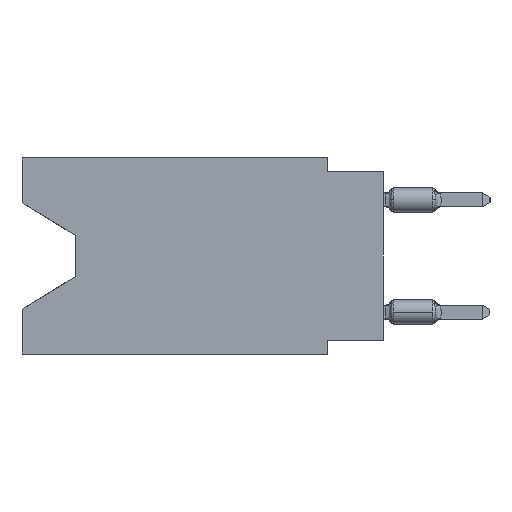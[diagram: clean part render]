
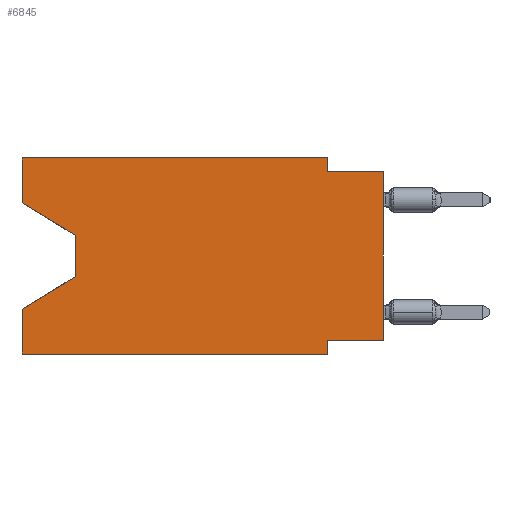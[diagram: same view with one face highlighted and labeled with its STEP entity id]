
A CAD part, left-side view. The second image highlights one B-rep face of the part: STEP entity #6845.
In plain terms, the highlighted planar face has unit normal (-1, 0, 0).
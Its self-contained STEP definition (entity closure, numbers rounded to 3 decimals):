
#188 = CARTESIAN_POINT ( 'NONE',  ( 0., 16.383, 0. ) ) ;
#1054 = CARTESIAN_POINT ( 'NONE',  ( 0., 2.54, 0. ) ) ;
#1588 = VERTEX_POINT ( 'NONE', #1054 ) ;
#1661 = VERTEX_POINT ( 'NONE', #5402 ) ;
#2791 = DIRECTION ( 'NONE',  ( 0., 0., 1. ) ) ;
#3307 = CARTESIAN_POINT ( 'NONE',  ( 0., 16.383, 0. ) ) ;
#3819 = LINE ( 'NONE', #188, #11470 ) ;
#4029 = CARTESIAN_POINT ( 'NONE',  ( 0., 16.383, 0. ) ) ;
#5402 = CARTESIAN_POINT ( 'NONE',  ( 0., 16.383, -8.89 ) ) ;
#5623 = CARTESIAN_POINT ( 'NONE',  ( 0., 16.383, -6.852 ) ) ;
#6257 = EDGE_CURVE ( 'NONE', #7869, #8992, #46836, .T. ) ;
#6414 = CARTESIAN_POINT ( 'NONE',  ( 0., 13.97, -5.385 ) ) ;
#6783 = DIRECTION ( 'NONE',  ( 0., 0., 1. ) ) ;
#6845 = ADVANCED_FACE ( 'NONE', ( #30512 ), #23268, .F. ) ;
#7869 = VERTEX_POINT ( 'NONE', #35128 ) ;
#8992 = VERTEX_POINT ( 'NONE', #31027 ) ;
#9885 = EDGE_LOOP ( 'NONE', ( #32290, #25213, #33541, #35533, #13075, #37361, #36365, #41042, #34936, #41778, #25624, #45189 ) ) ;
#9987 = EDGE_CURVE ( 'NONE', #44890, #39146, #24137, .T. ) ;
#10009 = VECTOR ( 'NONE', #6783, 1000. ) ;
#10449 = EDGE_CURVE ( 'NONE', #46667, #24446, #29289, .T. ) ;
#10716 = CARTESIAN_POINT ( 'NONE',  ( 0., 13.97, -5.385 ) ) ;
#11265 = DIRECTION ( 'NONE',  ( 0., -1., 0. ) ) ;
#11385 = DIRECTION ( 'NONE',  ( 0., -0.855, -0.519 ) ) ;
#11470 = VECTOR ( 'NONE', #14944, 1000. ) ;
#11976 = DIRECTION ( 'NONE',  ( 0., 0., -1. ) ) ;
#12849 = CARTESIAN_POINT ( 'NONE',  ( 0., 0., -8.255 ) ) ;
#13075 = ORIENTED_EDGE ( 'NONE', *, *, #45342, .T. ) ;
#13624 = DIRECTION ( 'NONE',  ( 0., 1., 0. ) ) ;
#14944 = DIRECTION ( 'NONE',  ( 0., 0., 1. ) ) ;
#15342 = DIRECTION ( 'NONE',  ( 0., 0., -1. ) ) ;
#16228 = CARTESIAN_POINT ( 'NONE',  ( 0., 16.383, 0. ) ) ;
#17009 = VERTEX_POINT ( 'NONE', #6414 ) ;
#17662 = VECTOR ( 'NONE', #15342, 1000. ) ;
#19204 = LINE ( 'NONE', #33989, #17662 ) ;
#20173 = LINE ( 'NONE', #21131, #23762 ) ;
#20389 = VERTEX_POINT ( 'NONE', #12849 ) ;
#20493 = DIRECTION ( 'NONE',  ( 0., 0., -1. ) ) ;
#20900 = CARTESIAN_POINT ( 'NONE',  ( 0., 2.54, -8.89 ) ) ;
#21131 = CARTESIAN_POINT ( 'NONE',  ( 0., 0., -8.255 ) ) ;
#21434 = EDGE_CURVE ( 'NONE', #20389, #8992, #46630, .T. ) ;
#21644 = CARTESIAN_POINT ( 'NONE',  ( 0., 0., -0.635 ) ) ;
#22300 = VERTEX_POINT ( 'NONE', #5623 ) ;
#22898 = EDGE_CURVE ( 'NONE', #24446, #17009, #30377, .T. ) ;
#23268 = PLANE ( 'NONE',  #43030 ) ;
#23762 = VECTOR ( 'NONE', #13624, 1000. ) ;
#24137 = LINE ( 'NONE', #38889, #39301 ) ;
#24311 = DIRECTION ( 'NONE',  ( 0., -1., 0. ) ) ;
#24446 = VERTEX_POINT ( 'NONE', #38228 ) ;
#25213 = ORIENTED_EDGE ( 'NONE', *, *, #22898, .T. ) ;
#25624 = ORIENTED_EDGE ( 'NONE', *, *, #26210, .F. ) ;
#26145 = CARTESIAN_POINT ( 'NONE',  ( 0., 16.383, -2.038 ) ) ;
#26210 = EDGE_CURVE ( 'NONE', #42825, #1588, #47594, .T. ) ;
#26368 = VECTOR ( 'NONE', #29830, 1000. ) ;
#26644 = DIRECTION ( 'NONE',  ( 1., 0., 0. ) ) ;
#27123 = DIRECTION ( 'NONE',  ( 0., 0., -1. ) ) ;
#28394 = VECTOR ( 'NONE', #46257, 1000. ) ;
#28519 = VECTOR ( 'NONE', #11385, 1000. ) ;
#29289 = LINE ( 'NONE', #26145, #28519 ) ;
#29520 = CARTESIAN_POINT ( 'NONE',  ( 0., 16.383, -2.038 ) ) ;
#29830 = DIRECTION ( 'NONE',  ( 0., 0.855, -0.519 ) ) ;
#30377 = LINE ( 'NONE', #45147, #45670 ) ;
#30512 = FACE_OUTER_BOUND ( 'NONE', #9885, .T. ) ;
#31027 = CARTESIAN_POINT ( 'NONE',  ( 0., 0., -0.635 ) ) ;
#31958 = LINE ( 'NONE', #35825, #28394 ) ;
#32290 = ORIENTED_EDGE ( 'NONE', *, *, #10449, .T. ) ;
#32413 = VECTOR ( 'NONE', #2791, 1000. ) ;
#33161 = VECTOR ( 'NONE', #24311, 1000. ) ;
#33541 = ORIENTED_EDGE ( 'NONE', *, *, #40415, .T. ) ;
#33989 = CARTESIAN_POINT ( 'NONE',  ( 0., 2.54, 0. ) ) ;
#34936 = ORIENTED_EDGE ( 'NONE', *, *, #6257, .F. ) ;
#35038 = EDGE_CURVE ( 'NONE', #20389, #44890, #20173, .T. ) ;
#35128 = CARTESIAN_POINT ( 'NONE',  ( 0., 2.54, -0.635 ) ) ;
#35533 = ORIENTED_EDGE ( 'NONE', *, *, #46722, .F. ) ;
#35825 = CARTESIAN_POINT ( 'NONE',  ( 0., 16.383, -8.89 ) ) ;
#36365 = ORIENTED_EDGE ( 'NONE', *, *, #35038, .F. ) ;
#37361 = ORIENTED_EDGE ( 'NONE', *, *, #9987, .F. ) ;
#37362 = EDGE_CURVE ( 'NONE', #46667, #42825, #3819, .T. ) ;
#38228 = CARTESIAN_POINT ( 'NONE',  ( 0., 13.97, -3.505 ) ) ;
#38889 = CARTESIAN_POINT ( 'NONE',  ( 0., 2.54, -8.89 ) ) ;
#39146 = VERTEX_POINT ( 'NONE', #20900 ) ;
#39301 = VECTOR ( 'NONE', #20493, 1000. ) ;
#39693 = LINE ( 'NONE', #44044, #10009 ) ;
#40415 = EDGE_CURVE ( 'NONE', #17009, #22300, #43863, .T. ) ;
#41042 = ORIENTED_EDGE ( 'NONE', *, *, #21434, .T. ) ;
#41094 = VECTOR ( 'NONE', #11265, 1000. ) ;
#41778 = ORIENTED_EDGE ( 'NONE', *, *, #44643, .F. ) ;
#42825 = VERTEX_POINT ( 'NONE', #3307 ) ;
#42974 = CARTESIAN_POINT ( 'NONE',  ( 0., 0., 0. ) ) ;
#43030 = AXIS2_PLACEMENT_3D ( 'NONE', #16228, #26644, #27123 ) ;
#43140 = CARTESIAN_POINT ( 'NONE',  ( 0., 2.54, -8.255 ) ) ;
#43863 = LINE ( 'NONE', #10716, #26368 ) ;
#44044 = CARTESIAN_POINT ( 'NONE',  ( 0., 16.383, 0. ) ) ;
#44643 = EDGE_CURVE ( 'NONE', #1588, #7869, #19204, .T. ) ;
#44890 = VERTEX_POINT ( 'NONE', #43140 ) ;
#45147 = CARTESIAN_POINT ( 'NONE',  ( 0., 13.97, -3.505 ) ) ;
#45189 = ORIENTED_EDGE ( 'NONE', *, *, #37362, .F. ) ;
#45342 = EDGE_CURVE ( 'NONE', #1661, #39146, #31958, .T. ) ;
#45670 = VECTOR ( 'NONE', #11976, 1000. ) ;
#46257 = DIRECTION ( 'NONE',  ( 0., -1., 0. ) ) ;
#46630 = LINE ( 'NONE', #42974, #32413 ) ;
#46667 = VERTEX_POINT ( 'NONE', #29520 ) ;
#46722 = EDGE_CURVE ( 'NONE', #1661, #22300, #39693, .T. ) ;
#46836 = LINE ( 'NONE', #21644, #33161 ) ;
#47594 = LINE ( 'NONE', #4029, #41094 ) ;
